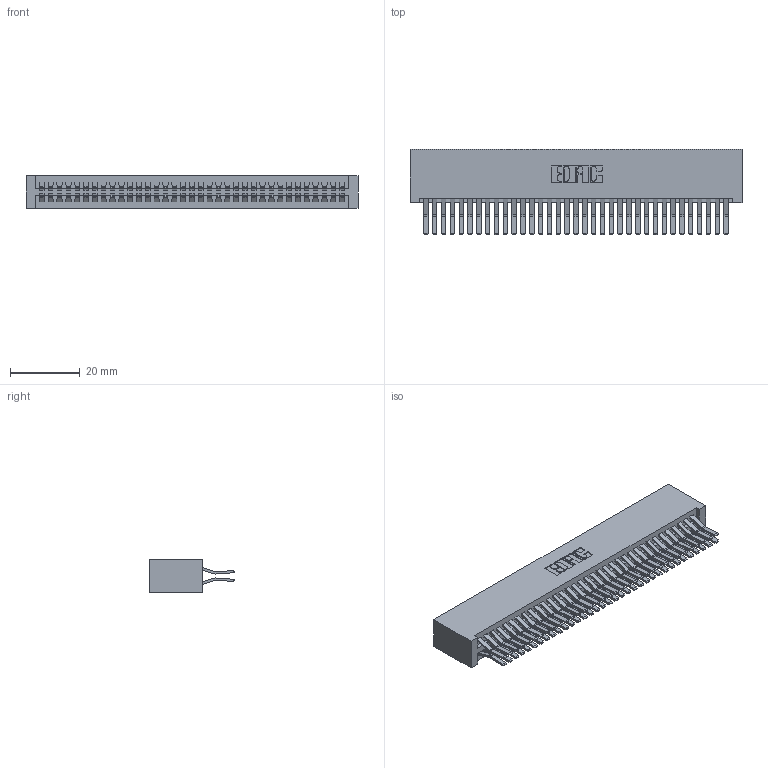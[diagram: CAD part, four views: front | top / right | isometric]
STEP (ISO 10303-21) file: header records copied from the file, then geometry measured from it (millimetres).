
FILE_DESCRIPTION (( 'STEP AP203' ), '1' );
FILE_NAME ('395-070-560-201.STEP', '2019-10-24T11:21:57', ( '' ), ( '' ), 'SwSTEP 2.0', 'SolidWorks 2016', '' );
FILE_SCHEMA (( 'CONFIG_CONTROL_DESIGN' ));
Length unit declared in the file: inch
Products named in the file (3): 345 Part_No Mounting Lugs; 345-292-001_560 Tail; 395-070-560-201
Assembly tree (71 placements, depth 2):
  395-070-560-201
    345 Part_No Mounting Lugs
    345-292-001_560 Tail  x70
Bounding box: 95.5 x 24.45 x 9.4 mm (x, y, z)
Volume: 10287.1 mm3; surface area: 16553.8 mm2
Topology: 71 solids, 71 shells, 3758 faces, 11167 edges, 7350 vertices
Faces by surface type: plane 2386, cylinder 1372
Entity records: 28215 total; most frequent: CARTESIAN_POINT 4736, ORIENTED_EDGE 4670, DIRECTION 4183, EDGE_CURVE 2335, VECTOR 2067, LINE 2067, VERTEX_POINT 1554, AXIS2_PLACEMENT_3D 1058
